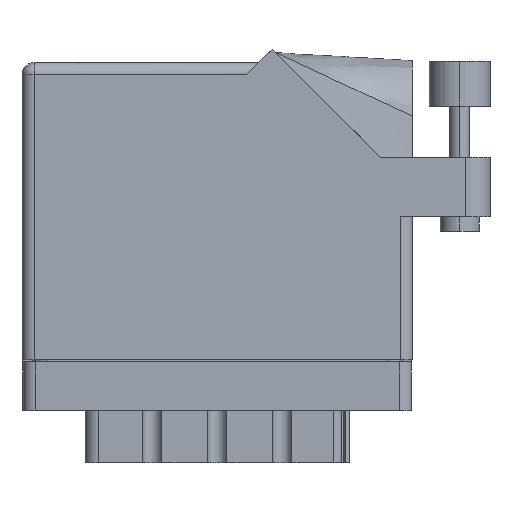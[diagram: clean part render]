
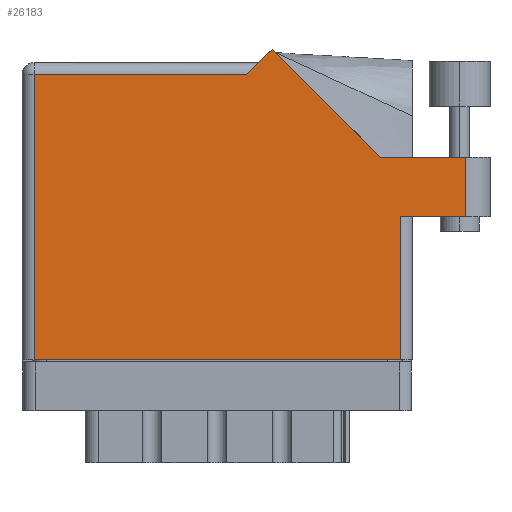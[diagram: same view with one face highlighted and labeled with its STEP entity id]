
A CAD part, front view. The second image highlights one B-rep face of the part: STEP entity #26183.
In plain terms, the highlighted face is planar.
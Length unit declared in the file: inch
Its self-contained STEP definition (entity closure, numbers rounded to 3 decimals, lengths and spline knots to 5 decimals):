
#412 = VECTOR ( 'NONE', #35591, 39.37008 ) ;
#936 = CARTESIAN_POINT ( 'NONE',  ( 2.01, 0.737, 0. ) ) ;
#940 = CARTESIAN_POINT ( 'NONE',  ( 0.062, 0., 0. ) ) ;
#1531 = ORIENTED_EDGE ( 'NONE', *, *, #17852, .T. ) ;
#2345 = CARTESIAN_POINT ( 'NONE',  ( 1.948, 0.737, 0. ) ) ;
#2871 = DIRECTION ( 'NONE',  ( 0., 0., -1. ) ) ;
#2959 = CARTESIAN_POINT ( 'NONE',  ( 2.41, 1.044, 0. ) ) ;
#3029 = ORIENTED_EDGE ( 'NONE', *, *, #5002, .T. ) ;
#3407 = EDGE_CURVE ( 'NONE', #8980, #19607, #13034, .T. ) ;
#3463 = DIRECTION ( 'NONE',  ( 1., 0., 0. ) ) ;
#3839 = EDGE_CURVE ( 'NONE', #19607, #5064, #15704, .T. ) ;
#4367 = ORIENTED_EDGE ( 'NONE', *, *, #31904, .T. ) ;
#4900 = CARTESIAN_POINT ( 'NONE',  ( 1.84442, 1.044, 0. ) ) ;
#5002 = EDGE_CURVE ( 'NONE', #5900, #7509, #30455, .T. ) ;
#5023 = CARTESIAN_POINT ( 'NONE',  ( 0.062, 1.468, 0. ) ) ;
#5064 = VERTEX_POINT ( 'NONE', #14885 ) ;
#5518 = CARTESIAN_POINT ( 'NONE',  ( 0., 0., 0. ) ) ;
#5757 = CARTESIAN_POINT ( 'NONE',  ( 0.062, 0., 0. ) ) ;
#5900 = VERTEX_POINT ( 'NONE', #5023 ) ;
#6760 = AXIS2_PLACEMENT_3D ( 'NONE', #19858, #2871, #22735 ) ;
#7065 = VECTOR ( 'NONE', #10104, 39.37008 ) ;
#7249 = LINE ( 'NONE', #2959, #12651 ) ;
#7509 = VERTEX_POINT ( 'NONE', #940 ) ;
#8980 = VERTEX_POINT ( 'NONE', #9277 ) ;
#9277 = CARTESIAN_POINT ( 'NONE',  ( 1.84442, 1.044, 0. ) ) ;
#9286 = LINE ( 'NONE', #5518, #11971 ) ;
#10104 = DIRECTION ( 'NONE',  ( -1., 0., 0. ) ) ;
#10247 = VERTEX_POINT ( 'NONE', #19999 ) ;
#11680 = DIRECTION ( 'NONE',  ( 0., 1., 0. ) ) ;
#11971 = VECTOR ( 'NONE', #37392, 39.37008 ) ;
#12651 = VECTOR ( 'NONE', #19939, 39.37008 ) ;
#12724 = CARTESIAN_POINT ( 'NONE',  ( 0., 1.468, 0. ) ) ;
#12810 = VECTOR ( 'NONE', #11680, 39.37008 ) ;
#13034 = LINE ( 'NONE', #4900, #23816 ) ;
#14885 = CARTESIAN_POINT ( 'NONE',  ( 1.155, 1.468, 0. ) ) ;
#15704 = LINE ( 'NONE', #29777, #412 ) ;
#16254 = FACE_OUTER_BOUND ( 'NONE', #29236, .T. ) ;
#16844 = PLANE ( 'NONE',  #6760 ) ;
#17852 = EDGE_CURVE ( 'NONE', #26662, #22037, #36532, .T. ) ;
#18872 = ORIENTED_EDGE ( 'NONE', *, *, #24220, .T. ) ;
#19607 = VERTEX_POINT ( 'NONE', #37078 ) ;
#19858 = CARTESIAN_POINT ( 'NONE',  ( 0., 1.53, 0. ) ) ;
#19939 = DIRECTION ( 'NONE',  ( -1., 0., 0. ) ) ;
#19999 = CARTESIAN_POINT ( 'NONE',  ( 2.285, 1.044, 0. ) ) ;
#20750 = VECTOR ( 'NONE', #3463, 39.37008 ) ;
#21080 = EDGE_CURVE ( 'NONE', #5064, #5900, #29120, .T. ) ;
#21845 = EDGE_CURVE ( 'NONE', #7509, #32600, #9286, .T. ) ;
#22037 = VERTEX_POINT ( 'NONE', #32637 ) ;
#22377 = ORIENTED_EDGE ( 'NONE', *, *, #3839, .T. ) ;
#22735 = DIRECTION ( 'NONE',  ( -1., 0., 0. ) ) ;
#22774 = EDGE_CURVE ( 'NONE', #32600, #26662, #27610, .T. ) ;
#23816 = VECTOR ( 'NONE', #36241, 39.37008 ) ;
#24220 = EDGE_CURVE ( 'NONE', #22037, #10247, #25407, .T. ) ;
#24805 = CARTESIAN_POINT ( 'NONE',  ( 1.948, 0.737, 0. ) ) ;
#24884 = VECTOR ( 'NONE', #36813, 39.37008 ) ;
#25407 = LINE ( 'NONE', #28894, #12810 ) ;
#26183 = ADVANCED_FACE ( 'NONE', ( #16254 ), #16844, .F. ) ;
#26662 = VERTEX_POINT ( 'NONE', #2345 ) ;
#27610 = LINE ( 'NONE', #24805, #24884 ) ;
#28144 = DIRECTION ( 'NONE',  ( 0., -1., 0. ) ) ;
#28894 = CARTESIAN_POINT ( 'NONE',  ( 2.285, 1.044, 0. ) ) ;
#29120 = LINE ( 'NONE', #12724, #7065 ) ;
#29236 = EDGE_LOOP ( 'NONE', ( #1531, #18872, #4367, #34086, #22377, #29889, #3029, #34805, #34387 ) ) ;
#29777 = CARTESIAN_POINT ( 'NONE',  ( 1.217, 1.53, 0. ) ) ;
#29889 = ORIENTED_EDGE ( 'NONE', *, *, #21080, .T. ) ;
#30455 = LINE ( 'NONE', #5757, #33628 ) ;
#31904 = EDGE_CURVE ( 'NONE', #10247, #8980, #7249, .T. ) ;
#31981 = CARTESIAN_POINT ( 'NONE',  ( 1.948, 0., 0. ) ) ;
#32600 = VERTEX_POINT ( 'NONE', #31981 ) ;
#32637 = CARTESIAN_POINT ( 'NONE',  ( 2.285, 0.737, 0. ) ) ;
#33628 = VECTOR ( 'NONE', #28144, 39.37008 ) ;
#34086 = ORIENTED_EDGE ( 'NONE', *, *, #3407, .T. ) ;
#34387 = ORIENTED_EDGE ( 'NONE', *, *, #22774, .T. ) ;
#34805 = ORIENTED_EDGE ( 'NONE', *, *, #21845, .T. ) ;
#35591 = DIRECTION ( 'NONE',  ( -0.707, -0.707, 0. ) ) ;
#36241 = DIRECTION ( 'NONE',  ( -0.707, 0.707, 0. ) ) ;
#36532 = LINE ( 'NONE', #936, #20750 ) ;
#36813 = DIRECTION ( 'NONE',  ( 0., 1., 0. ) ) ;
#37078 = CARTESIAN_POINT ( 'NONE',  ( 1.28771, 1.60071, 0. ) ) ;
#37392 = DIRECTION ( 'NONE',  ( 1., 0., 0. ) ) ;
